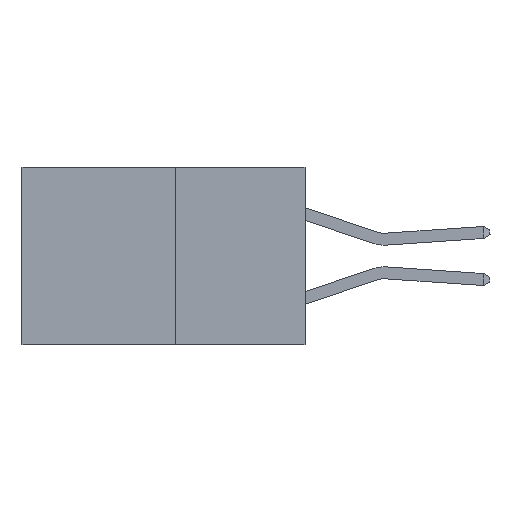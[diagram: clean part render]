
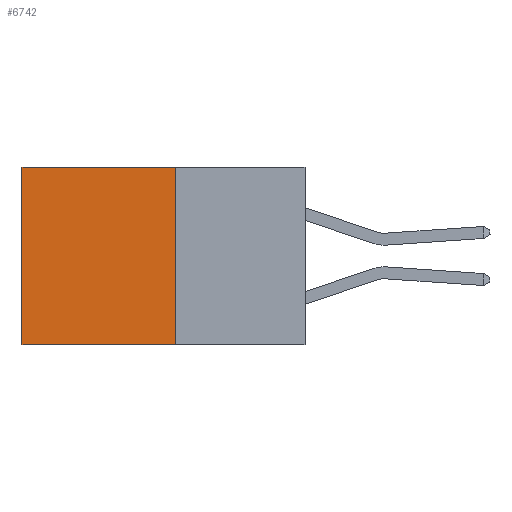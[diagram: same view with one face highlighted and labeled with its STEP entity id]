
A CAD part, left-side view. The second image highlights one B-rep face of the part: STEP entity #6742.
In plain terms, the highlighted planar face has unit normal (-1, 0, 0).
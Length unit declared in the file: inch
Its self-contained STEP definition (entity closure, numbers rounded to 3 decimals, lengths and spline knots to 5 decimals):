
#1015 = CARTESIAN_POINT ( 'NONE',  ( 0.277, 0.27, 0. ) ) ;
#1344 = ORIENTED_EDGE ( 'NONE', *, *, #5966, .F. ) ;
#1638 = ORIENTED_EDGE ( 'NONE', *, *, #16231, .T. ) ;
#1831 = CARTESIAN_POINT ( 'NONE',  ( 0.277, 0.59, 0. ) ) ;
#2217 = LINE ( 'NONE', #1015, #8661 ) ;
#3281 = EDGE_LOOP ( 'NONE', ( #15389, #21167, #1344, #1638 ) ) ;
#4851 = EDGE_CURVE ( 'NONE', #15033, #8399, #17511, .T. ) ;
#5966 = EDGE_CURVE ( 'NONE', #10099, #30655, #12121, .T. ) ;
#6742 = ADVANCED_FACE ( 'NONE', ( #23086 ), #30976, .F. ) ;
#8196 = DIRECTION ( 'NONE',  ( 0., 0., -1. ) ) ;
#8399 = VERTEX_POINT ( 'NONE', #13499 ) ;
#8661 = VECTOR ( 'NONE', #10642, 39.37008 ) ;
#10099 = VERTEX_POINT ( 'NONE', #14467 ) ;
#10642 = DIRECTION ( 'NONE',  ( 0., 1., 0. ) ) ;
#11071 = VECTOR ( 'NONE', #29095, 39.37008 ) ;
#11221 = CARTESIAN_POINT ( 'NONE',  ( 0.277, 0.27, -0.37 ) ) ;
#11538 = CARTESIAN_POINT ( 'NONE',  ( 0.277, 0.59, -0.37 ) ) ;
#12121 = LINE ( 'NONE', #11221, #24255 ) ;
#13499 = CARTESIAN_POINT ( 'NONE',  ( 0.277, 0.59, -0.37 ) ) ;
#14467 = CARTESIAN_POINT ( 'NONE',  ( 0.277, 0.27, 0. ) ) ;
#15033 = VERTEX_POINT ( 'NONE', #1831 ) ;
#15389 = ORIENTED_EDGE ( 'NONE', *, *, #4851, .T. ) ;
#16231 = EDGE_CURVE ( 'NONE', #10099, #15033, #2217, .T. ) ;
#17201 = DIRECTION ( 'NONE',  ( 0., 1., 0. ) ) ;
#17511 = LINE ( 'NONE', #11538, #11071 ) ;
#18104 = AXIS2_PLACEMENT_3D ( 'NONE', #31001, #30672, #30593 ) ;
#19531 = CARTESIAN_POINT ( 'NONE',  ( 0.277, 0.27, -0.37 ) ) ;
#21167 = ORIENTED_EDGE ( 'NONE', *, *, #26279, .F. ) ;
#23086 = FACE_OUTER_BOUND ( 'NONE', #3281, .T. ) ;
#24255 = VECTOR ( 'NONE', #8196, 39.37008 ) ;
#26279 = EDGE_CURVE ( 'NONE', #30655, #8399, #30613, .T. ) ;
#27028 = CARTESIAN_POINT ( 'NONE',  ( 0.277, 0.27, -0.37 ) ) ;
#29095 = DIRECTION ( 'NONE',  ( 0., 0., -1. ) ) ;
#29858 = VECTOR ( 'NONE', #17201, 39.37008 ) ;
#30593 = DIRECTION ( 'NONE',  ( 0., 0., -1. ) ) ;
#30613 = LINE ( 'NONE', #19531, #29858 ) ;
#30655 = VERTEX_POINT ( 'NONE', #27028 ) ;
#30672 = DIRECTION ( 'NONE',  ( 1., 0., 0. ) ) ;
#30976 = PLANE ( 'NONE',  #18104 ) ;
#31001 = CARTESIAN_POINT ( 'NONE',  ( 0.277, 0.27, -0.37 ) ) ;
